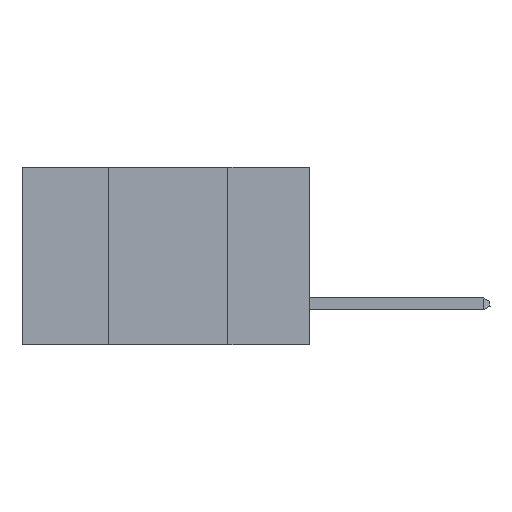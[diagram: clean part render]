
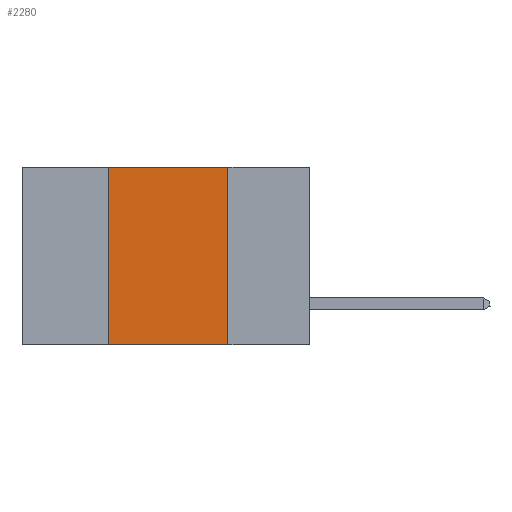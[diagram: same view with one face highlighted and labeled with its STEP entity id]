
A CAD part, left-side view. The second image highlights one B-rep face of the part: STEP entity #2280.
In plain terms, the highlighted planar face has unit normal (-1, 0, 0).
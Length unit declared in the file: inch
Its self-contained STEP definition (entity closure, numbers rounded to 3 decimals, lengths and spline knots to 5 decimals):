
#89 = CARTESIAN_POINT ( 'NONE',  ( 0., 0.42, 0. ) ) ;
#209 = VERTEX_POINT ( 'NONE', #4715 ) ;
#845 = VERTEX_POINT ( 'NONE', #12124 ) ;
#1532 = LINE ( 'NONE', #5427, #2111 ) ;
#1878 = DIRECTION ( 'NONE',  ( 0., 0., -1. ) ) ;
#1903 = ORIENTED_EDGE ( 'NONE', *, *, #7228, .F. ) ;
#2111 = VECTOR ( 'NONE', #7863, 39.37008 ) ;
#2280 = ADVANCED_FACE ( 'NONE', ( #7573 ), #5463, .F. ) ;
#2450 = DIRECTION ( 'NONE',  ( 0., 0., 1. ) ) ;
#2969 = VECTOR ( 'NONE', #2450, 39.37008 ) ;
#3485 = EDGE_CURVE ( 'NONE', #8907, #845, #14337, .T. ) ;
#3651 = LINE ( 'NONE', #14966, #10256 ) ;
#4284 = EDGE_LOOP ( 'NONE', ( #13234, #1903, #14980, #9802 ) ) ;
#4295 = AXIS2_PLACEMENT_3D ( 'NONE', #13926, #15138, #1878 ) ;
#4610 = EDGE_CURVE ( 'NONE', #8907, #209, #7851, .T. ) ;
#4715 = CARTESIAN_POINT ( 'NONE',  ( 0., 0.17, -0.37 ) ) ;
#5427 = CARTESIAN_POINT ( 'NONE',  ( 0., 0.17, 0. ) ) ;
#5463 = PLANE ( 'NONE',  #4295 ) ;
#7228 = EDGE_CURVE ( 'NONE', #845, #10613, #3651, .T. ) ;
#7383 = CARTESIAN_POINT ( 'NONE',  ( 0., 0.42, -0.37 ) ) ;
#7571 = EDGE_CURVE ( 'NONE', #10613, #209, #1532, .T. ) ;
#7573 = FACE_OUTER_BOUND ( 'NONE', #4284, .T. ) ;
#7851 = LINE ( 'NONE', #13981, #13536 ) ;
#7863 = DIRECTION ( 'NONE',  ( 0., 0., -1. ) ) ;
#8907 = VERTEX_POINT ( 'NONE', #7383 ) ;
#9802 = ORIENTED_EDGE ( 'NONE', *, *, #4610, .T. ) ;
#10256 = VECTOR ( 'NONE', #12601, 39.37008 ) ;
#10613 = VERTEX_POINT ( 'NONE', #13307 ) ;
#12124 = CARTESIAN_POINT ( 'NONE',  ( 0., 0.42, 0. ) ) ;
#12601 = DIRECTION ( 'NONE',  ( 0., -1., 0. ) ) ;
#13234 = ORIENTED_EDGE ( 'NONE', *, *, #7571, .F. ) ;
#13307 = CARTESIAN_POINT ( 'NONE',  ( 0., 0.17, 0. ) ) ;
#13536 = VECTOR ( 'NONE', #13876, 39.37008 ) ;
#13876 = DIRECTION ( 'NONE',  ( 0., -1., 0. ) ) ;
#13926 = CARTESIAN_POINT ( 'NONE',  ( 0., 0.6, 0. ) ) ;
#13981 = CARTESIAN_POINT ( 'NONE',  ( 0., 0.6, -0.37 ) ) ;
#14337 = LINE ( 'NONE', #89, #2969 ) ;
#14966 = CARTESIAN_POINT ( 'NONE',  ( 0., 0.6, 0. ) ) ;
#14980 = ORIENTED_EDGE ( 'NONE', *, *, #3485, .F. ) ;
#15138 = DIRECTION ( 'NONE',  ( 1., 0., 0. ) ) ;
